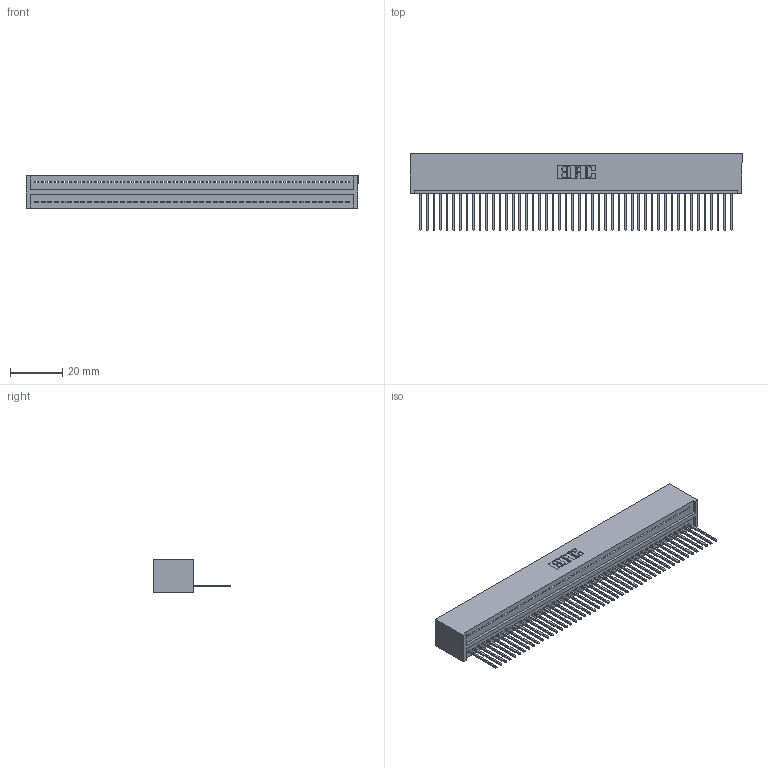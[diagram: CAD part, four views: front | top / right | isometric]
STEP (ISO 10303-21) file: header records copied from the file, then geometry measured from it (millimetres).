
FILE_DESCRIPTION (( 'STEP AP203' ), '1' );
FILE_NAME ('325-048-540-101.STEP', '2020-02-24T23:27:19', ( '' ), ( '' ), 'SwSTEP 2.0', 'SolidWorks 2016', '' );
FILE_SCHEMA (( 'CONFIG_CONTROL_DESIGN' ));
Length unit declared in the file: inch
Products named in the file (3): 325-048-540-101; 325 Part_Lugless; 325-292-001_325-293-140
Assembly tree (49 placements, depth 2):
  325-048-540-101
    325 Part_Lugless
    325-292-001_325-293-140  x48
Bounding box: 127.56 x 29.46 x 12.45 mm (x, y, z)
Volume: 16877.7 mm3; surface area: 19511.8 mm2
Topology: 49 solids, 49 shells, 2890 faces, 8735 edges, 5758 vertices
Faces by surface type: plane 2082, cylinder 808
Entity records: 28309 total; most frequent: CARTESIAN_POINT 4890, ORIENTED_EDGE 4874, DIRECTION 4105, EDGE_CURVE 2437, VECTOR 2317, LINE 2317, VERTEX_POINT 1622, AXIS2_PLACEMENT_3D 894
